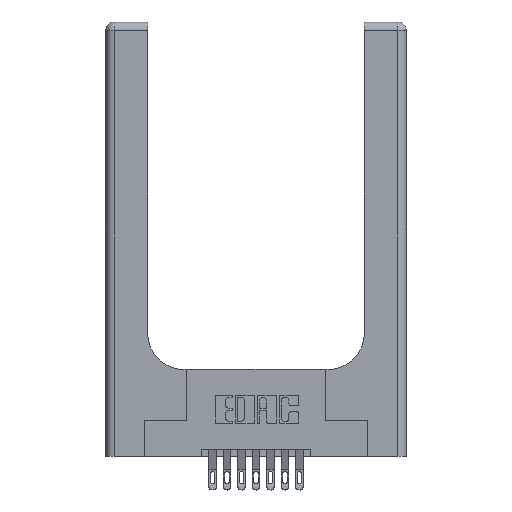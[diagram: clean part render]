
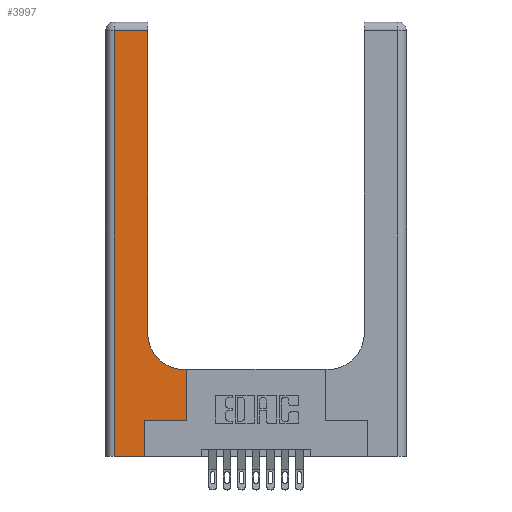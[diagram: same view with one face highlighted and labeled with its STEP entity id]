
A CAD part, top view. The second image highlights one B-rep face of the part: STEP entity #3997.
In plain terms, the highlighted planar face has unit normal (0, 0, 1).
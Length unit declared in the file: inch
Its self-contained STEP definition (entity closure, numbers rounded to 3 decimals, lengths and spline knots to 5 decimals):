
#80 = VECTOR ( 'NONE', #11440, 39.37008 ) ;
#1006 = EDGE_CURVE ( 'NONE', #9217, #13341, #12348, .T. ) ;
#1081 = LINE ( 'NONE', #15598, #13994 ) ;
#1111 = CARTESIAN_POINT ( 'NONE',  ( 0.269, 0.25, 0.37 ) ) ;
#1239 = CARTESIAN_POINT ( 'NONE',  ( 0., 0., 0.37 ) ) ;
#1644 = PLANE ( 'NONE',  #3293 ) ;
#1780 = FACE_OUTER_BOUND ( 'NONE', #7516, .T. ) ;
#1822 = CARTESIAN_POINT ( 'NONE',  ( 0.269, 0.25, 0.37 ) ) ;
#2126 = CARTESIAN_POINT ( 'NONE',  ( 0.5415, 0.85, 0.37 ) ) ;
#2454 = DIRECTION ( 'NONE',  ( 0., 1., 0. ) ) ;
#2726 = CARTESIAN_POINT ( 'NONE',  ( 0.5585, 0.25, 0.37 ) ) ;
#2936 = EDGE_CURVE ( 'NONE', #11283, #15064, #6515, .T. ) ;
#2970 = LINE ( 'NONE', #1111, #8672 ) ;
#3200 = DIRECTION ( 'NONE',  ( 0., -1., 0. ) ) ;
#3272 = VECTOR ( 'NONE', #3200, 39.37008 ) ;
#3293 = AXIS2_PLACEMENT_3D ( 'NONE', #4783, #4001, #3982 ) ;
#3349 = DIRECTION ( 'NONE',  ( 1., 0., 0. ) ) ;
#3453 = ORIENTED_EDGE ( 'NONE', *, *, #2936, .T. ) ;
#3759 = VECTOR ( 'NONE', #2454, 39.37008 ) ;
#3857 = EDGE_CURVE ( 'NONE', #7615, #11690, #6861, .T. ) ;
#3982 = DIRECTION ( 'NONE',  ( -1., 0., 0. ) ) ;
#3997 = ADVANCED_FACE ( 'NONE', ( #1780 ), #1644, .F. ) ;
#4001 = DIRECTION ( 'NONE',  ( 0., 0., -1. ) ) ;
#4190 = CARTESIAN_POINT ( 'NONE',  ( 0.5415, 0.6, 0.37 ) ) ;
#4191 = ORIENTED_EDGE ( 'NONE', *, *, #6314, .T. ) ;
#4324 = ORIENTED_EDGE ( 'NONE', *, *, #10323, .T. ) ;
#4783 = CARTESIAN_POINT ( 'NONE',  ( 0., 3., 0.37 ) ) ;
#4899 = DIRECTION ( 'NONE',  ( -1., 0., 0. ) ) ;
#4972 = CARTESIAN_POINT ( 'NONE',  ( 0., 2.94, 0.37 ) ) ;
#5433 = ORIENTED_EDGE ( 'NONE', *, *, #1006, .T. ) ;
#5659 = EDGE_CURVE ( 'NONE', #11690, #13565, #12991, .T. ) ;
#6314 = EDGE_CURVE ( 'NONE', #15064, #15421, #13917, .T. ) ;
#6515 = LINE ( 'NONE', #15602, #80 ) ;
#6861 = LINE ( 'NONE', #4972, #13018 ) ;
#6941 = CARTESIAN_POINT ( 'NONE',  ( 0.5585, 0.6, 0.37 ) ) ;
#7146 = ORIENTED_EDGE ( 'NONE', *, *, #11968, .T. ) ;
#7282 = CARTESIAN_POINT ( 'NONE',  ( 0.06, 0., 0.37 ) ) ;
#7516 = EDGE_LOOP ( 'NONE', ( #7146, #9449, #8293, #12328, #5433, #8868, #4324, #3453, #4191 ) ) ;
#7615 = VERTEX_POINT ( 'NONE', #8899 ) ;
#7802 = CARTESIAN_POINT ( 'NONE',  ( 0.06, 2.94, 0.37 ) ) ;
#8293 = ORIENTED_EDGE ( 'NONE', *, *, #5659, .T. ) ;
#8312 = DIRECTION ( 'NONE',  ( 0., 1., 0. ) ) ;
#8396 = DIRECTION ( 'NONE',  ( 0., 1., 0. ) ) ;
#8448 = CARTESIAN_POINT ( 'NONE',  ( 0.269, 0., 0.37 ) ) ;
#8672 = VECTOR ( 'NONE', #12063, 39.37008 ) ;
#8801 = LINE ( 'NONE', #1239, #11660 ) ;
#8868 = ORIENTED_EDGE ( 'NONE', *, *, #11398, .T. ) ;
#8899 = CARTESIAN_POINT ( 'NONE',  ( 0.2915, 2.94, 0.37 ) ) ;
#9086 = VECTOR ( 'NONE', #8312, 39.37008 ) ;
#9217 = VERTEX_POINT ( 'NONE', #9922 ) ;
#9449 = ORIENTED_EDGE ( 'NONE', *, *, #3857, .T. ) ;
#9858 = LINE ( 'NONE', #10964, #3759 ) ;
#9922 = CARTESIAN_POINT ( 'NONE',  ( 0.269, 0., 0.37 ) ) ;
#10323 = EDGE_CURVE ( 'NONE', #11617, #11283, #9858, .T. ) ;
#10632 = DIRECTION ( 'NONE',  ( 0., 0., -1. ) ) ;
#10964 = CARTESIAN_POINT ( 'NONE',  ( 0.5585, 0.25, 0.37 ) ) ;
#11283 = VERTEX_POINT ( 'NONE', #6941 ) ;
#11398 = EDGE_CURVE ( 'NONE', #13341, #11617, #2970, .T. ) ;
#11440 = DIRECTION ( 'NONE',  ( -1., 0., 0. ) ) ;
#11617 = VERTEX_POINT ( 'NONE', #2726 ) ;
#11660 = VECTOR ( 'NONE', #14147, 39.37008 ) ;
#11690 = VERTEX_POINT ( 'NONE', #7802 ) ;
#11968 = EDGE_CURVE ( 'NONE', #15421, #7615, #1081, .T. ) ;
#12063 = DIRECTION ( 'NONE',  ( 1., 0., 0. ) ) ;
#12172 = CARTESIAN_POINT ( 'NONE',  ( 0.2915, 0.85, 0.37 ) ) ;
#12328 = ORIENTED_EDGE ( 'NONE', *, *, #13558, .T. ) ;
#12348 = LINE ( 'NONE', #8448, #9086 ) ;
#12950 = CARTESIAN_POINT ( 'NONE',  ( 0.06, 3., 0.37 ) ) ;
#12991 = LINE ( 'NONE', #12950, #3272 ) ;
#13018 = VECTOR ( 'NONE', #4899, 39.37008 ) ;
#13341 = VERTEX_POINT ( 'NONE', #1822 ) ;
#13558 = EDGE_CURVE ( 'NONE', #13565, #9217, #8801, .T. ) ;
#13565 = VERTEX_POINT ( 'NONE', #7282 ) ;
#13917 = CIRCLE ( 'NONE', #15002, 0.25 ) ;
#13994 = VECTOR ( 'NONE', #8396, 39.37008 ) ;
#14147 = DIRECTION ( 'NONE',  ( 1., 0., 0. ) ) ;
#15002 = AXIS2_PLACEMENT_3D ( 'NONE', #2126, #10632, #3349 ) ;
#15064 = VERTEX_POINT ( 'NONE', #4190 ) ;
#15421 = VERTEX_POINT ( 'NONE', #12172 ) ;
#15598 = CARTESIAN_POINT ( 'NONE',  ( 0.2915, 3., 0.37 ) ) ;
#15602 = CARTESIAN_POINT ( 'NONE',  ( 0.2915, 0.6, 0.37 ) ) ;
